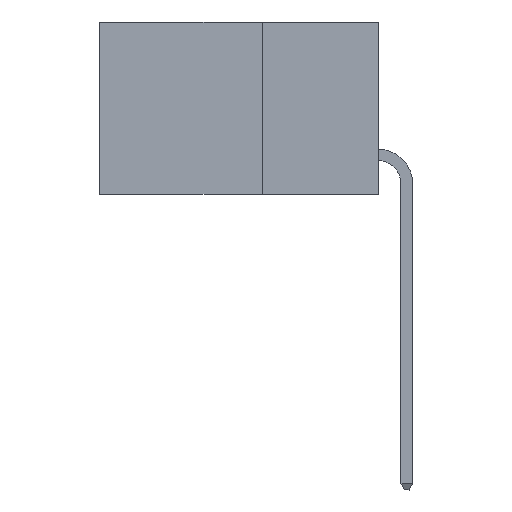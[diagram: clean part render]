
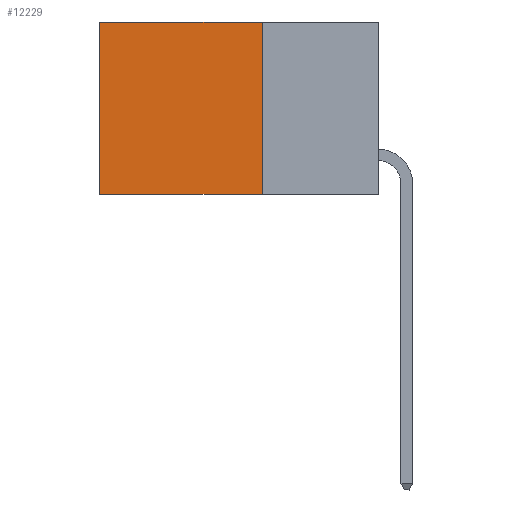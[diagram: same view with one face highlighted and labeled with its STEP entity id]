
A CAD part, left-side view. The second image highlights one B-rep face of the part: STEP entity #12229.
In plain terms, the highlighted planar face has unit normal (-1, 0, 0).
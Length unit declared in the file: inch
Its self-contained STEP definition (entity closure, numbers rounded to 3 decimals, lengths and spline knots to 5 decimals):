
#331 = VECTOR ( 'NONE', #12203, 39.37008 ) ;
#804 = VERTEX_POINT ( 'NONE', #2221 ) ;
#1213 = EDGE_CURVE ( 'NONE', #11831, #11533, #8491, .T. ) ;
#1329 = DIRECTION ( 'NONE',  ( 0., 0., -1. ) ) ;
#1484 = CARTESIAN_POINT ( 'NONE',  ( 0.2615, 0.25, -0.37 ) ) ;
#1543 = DIRECTION ( 'NONE',  ( 0., 0., -1. ) ) ;
#1591 = CARTESIAN_POINT ( 'NONE',  ( 0.2615, 0.25, -0.37 ) ) ;
#2221 = CARTESIAN_POINT ( 'NONE',  ( 0.2615, 0.6, 0. ) ) ;
#2379 = ORIENTED_EDGE ( 'NONE', *, *, #9315, .F. ) ;
#3771 = VECTOR ( 'NONE', #7844, 39.37008 ) ;
#4088 = ORIENTED_EDGE ( 'NONE', *, *, #1213, .F. ) ;
#4250 = CARTESIAN_POINT ( 'NONE',  ( 0.2615, 0.25, -0.37 ) ) ;
#4592 = CARTESIAN_POINT ( 'NONE',  ( 0.2615, 0.6, -0.37 ) ) ;
#5225 = CARTESIAN_POINT ( 'NONE',  ( 0.2615, 0.25, -0.37 ) ) ;
#5525 = LINE ( 'NONE', #4592, #5566 ) ;
#5566 = VECTOR ( 'NONE', #8434, 39.37008 ) ;
#5593 = ORIENTED_EDGE ( 'NONE', *, *, #8295, .T. ) ;
#5952 = ORIENTED_EDGE ( 'NONE', *, *, #11253, .T. ) ;
#7844 = DIRECTION ( 'NONE',  ( 0., 1., 0. ) ) ;
#7976 = CARTESIAN_POINT ( 'NONE',  ( 0.2615, 0.25, 0. ) ) ;
#8199 = DIRECTION ( 'NONE',  ( 1., 0., 0. ) ) ;
#8295 = EDGE_CURVE ( 'NONE', #804, #11533, #5525, .T. ) ;
#8434 = DIRECTION ( 'NONE',  ( 0., 0., -1. ) ) ;
#8491 = LINE ( 'NONE', #1591, #331 ) ;
#8969 = CARTESIAN_POINT ( 'NONE',  ( 0.2615, 0.25, 0. ) ) ;
#9315 = EDGE_CURVE ( 'NONE', #9795, #11831, #9961, .T. ) ;
#9572 = AXIS2_PLACEMENT_3D ( 'NONE', #1484, #8199, #1543 ) ;
#9795 = VERTEX_POINT ( 'NONE', #7976 ) ;
#9961 = LINE ( 'NONE', #5225, #10604 ) ;
#10005 = LINE ( 'NONE', #8969, #3771 ) ;
#10034 = FACE_OUTER_BOUND ( 'NONE', #10284, .T. ) ;
#10284 = EDGE_LOOP ( 'NONE', ( #5593, #4088, #2379, #5952 ) ) ;
#10604 = VECTOR ( 'NONE', #1329, 39.37008 ) ;
#11253 = EDGE_CURVE ( 'NONE', #9795, #804, #10005, .T. ) ;
#11533 = VERTEX_POINT ( 'NONE', #12508 ) ;
#11831 = VERTEX_POINT ( 'NONE', #4250 ) ;
#12023 = PLANE ( 'NONE',  #9572 ) ;
#12203 = DIRECTION ( 'NONE',  ( 0., 1., 0. ) ) ;
#12229 = ADVANCED_FACE ( 'NONE', ( #10034 ), #12023, .F. ) ;
#12508 = CARTESIAN_POINT ( 'NONE',  ( 0.2615, 0.6, -0.37 ) ) ;
